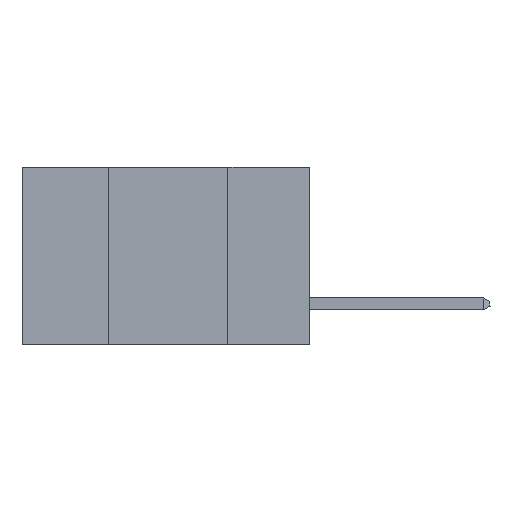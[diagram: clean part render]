
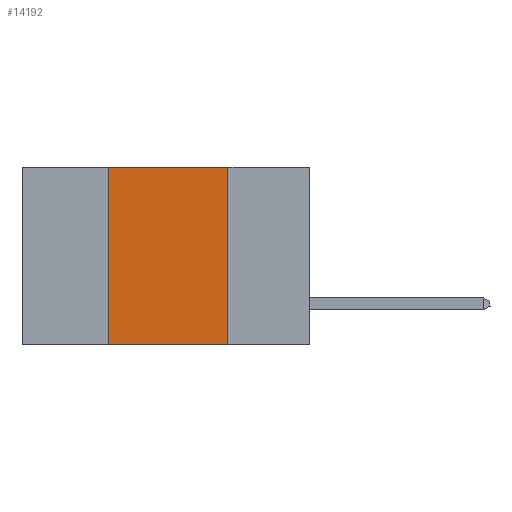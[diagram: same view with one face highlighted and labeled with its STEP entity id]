
A CAD part, left-side view. The second image highlights one B-rep face of the part: STEP entity #14192.
In plain terms, the highlighted planar face has unit normal (-1, 0, 0).
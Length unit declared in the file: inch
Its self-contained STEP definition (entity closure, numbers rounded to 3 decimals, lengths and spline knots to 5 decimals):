
#1064 = EDGE_CURVE ( 'NONE', #32391, #19475, #40626, .T. ) ;
#3510 = VECTOR ( 'NONE', #23009, 39.37008 ) ;
#6021 = LINE ( 'NONE', #11594, #3510 ) ;
#6349 = LINE ( 'NONE', #44455, #13163 ) ;
#6389 = EDGE_CURVE ( 'NONE', #27226, #48337, #6349, .T. ) ;
#6900 = DIRECTION ( 'NONE',  ( 0., 0., -1. ) ) ;
#8338 = EDGE_CURVE ( 'NONE', #19475, #48337, #42162, .T. ) ;
#10673 = ORIENTED_EDGE ( 'NONE', *, *, #34640, .F. ) ;
#11594 = CARTESIAN_POINT ( 'NONE',  ( 0., 0.42, 0. ) ) ;
#13163 = VECTOR ( 'NONE', #32234, 39.37008 ) ;
#13347 = FACE_OUTER_BOUND ( 'NONE', #14719, .T. ) ;
#14192 = ADVANCED_FACE ( 'NONE', ( #13347 ), #18985, .F. ) ;
#14719 = EDGE_LOOP ( 'NONE', ( #33701, #45643, #10673, #41148 ) ) ;
#17995 = CARTESIAN_POINT ( 'NONE',  ( 0., 0.17, 0. ) ) ;
#18199 = AXIS2_PLACEMENT_3D ( 'NONE', #38625, #23132, #42492 ) ;
#18985 = PLANE ( 'NONE',  #18199 ) ;
#19475 = VERTEX_POINT ( 'NONE', #17995 ) ;
#23009 = DIRECTION ( 'NONE',  ( 0., 0., 1. ) ) ;
#23132 = DIRECTION ( 'NONE',  ( 1., 0., 0. ) ) ;
#27226 = VERTEX_POINT ( 'NONE', #39691 ) ;
#30598 = VECTOR ( 'NONE', #31394, 39.37008 ) ;
#31394 = DIRECTION ( 'NONE',  ( 0., -1., 0. ) ) ;
#32234 = DIRECTION ( 'NONE',  ( 0., -1., 0. ) ) ;
#32391 = VERTEX_POINT ( 'NONE', #48311 ) ;
#33701 = ORIENTED_EDGE ( 'NONE', *, *, #8338, .F. ) ;
#34640 = EDGE_CURVE ( 'NONE', #27226, #32391, #6021, .T. ) ;
#35877 = VECTOR ( 'NONE', #6900, 39.37008 ) ;
#36140 = CARTESIAN_POINT ( 'NONE',  ( 0., 0.17, -0.37 ) ) ;
#38625 = CARTESIAN_POINT ( 'NONE',  ( 0., 0.6, 0. ) ) ;
#39600 = CARTESIAN_POINT ( 'NONE',  ( 0., 0.6, 0. ) ) ;
#39691 = CARTESIAN_POINT ( 'NONE',  ( 0., 0.42, -0.37 ) ) ;
#40626 = LINE ( 'NONE', #39600, #30598 ) ;
#41148 = ORIENTED_EDGE ( 'NONE', *, *, #6389, .T. ) ;
#42162 = LINE ( 'NONE', #50999, #35877 ) ;
#42492 = DIRECTION ( 'NONE',  ( 0., 0., -1. ) ) ;
#44455 = CARTESIAN_POINT ( 'NONE',  ( 0., 0.6, -0.37 ) ) ;
#45643 = ORIENTED_EDGE ( 'NONE', *, *, #1064, .F. ) ;
#48311 = CARTESIAN_POINT ( 'NONE',  ( 0., 0.42, 0. ) ) ;
#48337 = VERTEX_POINT ( 'NONE', #36140 ) ;
#50999 = CARTESIAN_POINT ( 'NONE',  ( 0., 0.17, 0. ) ) ;
